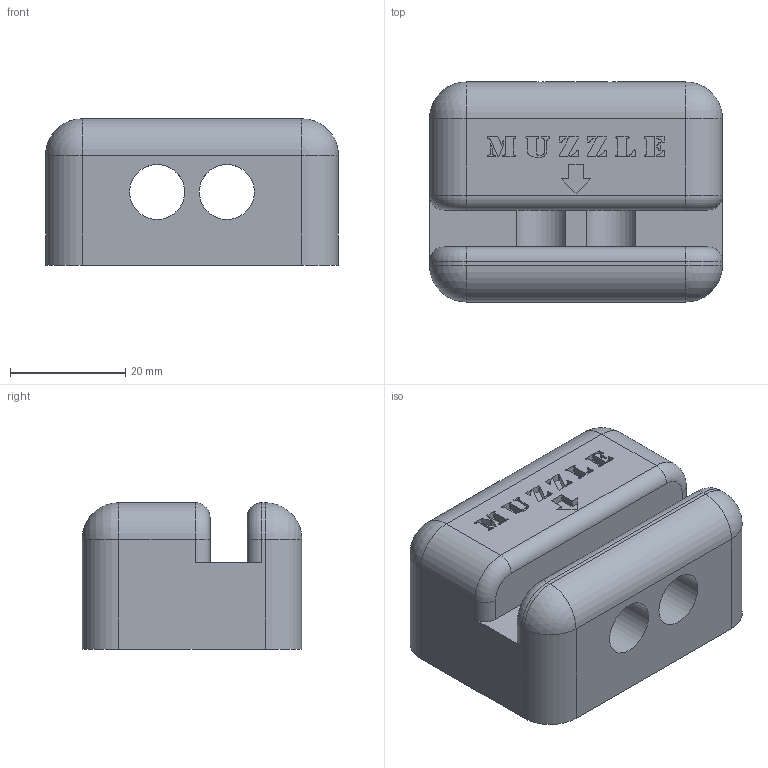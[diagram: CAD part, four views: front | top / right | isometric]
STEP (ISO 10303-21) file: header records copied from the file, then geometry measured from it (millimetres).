
FILE_DESCRIPTION (( 'STEP AP214' ), '1' );
FILE_NAME ('Notching_Guide.STEP', '2014-02-12T12:47:53', ( 'elpi' ), ( '' ), 'SwSTEP 2.0', 'SolidWorks 2013', '' );
FILE_SCHEMA (( 'AUTOMOTIVE_DESIGN' ));
Length unit declared in the file: inch
Products named in the file (1): Notching_Guide
Bounding box: 50.8 x 38.13 x 25.4 mm (x, y, z)
Volume: 38084.1 mm3; surface area: 10197.4 mm2
Topology: 1 solids, 1 shells, 252 faces, 682 edges, 440 vertices
Faces by surface type: bspline 108, plane 107, cylinder 18, torus 11, sphere 6, cone 2
Full cylindrical faces by diameter (mm): 9.55 x2
Entity records: 10656 total; most frequent: CARTESIAN_POINT 5045, ORIENTED_EDGE 1336, DIRECTION 807, EDGE_CURVE 668, VERTEX_POINT 436, VECTOR 383, LINE 383, EDGE_LOOP 278
